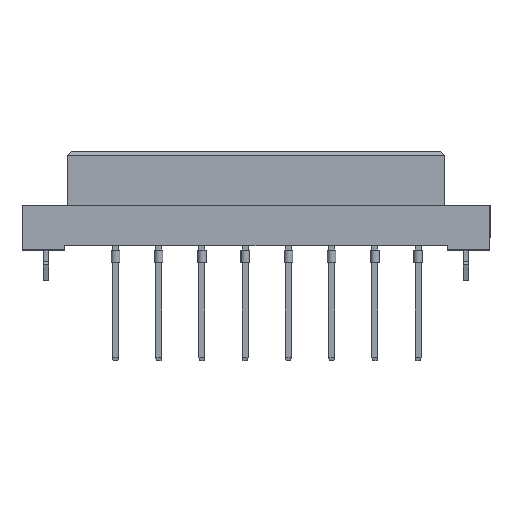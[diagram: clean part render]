
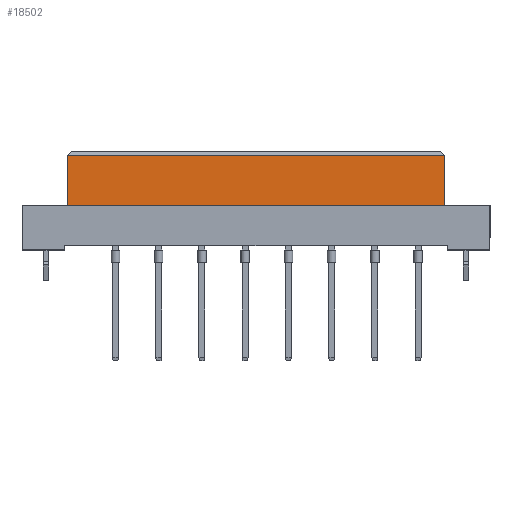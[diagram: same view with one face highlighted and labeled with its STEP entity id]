
A CAD part, top view. The second image highlights one B-rep face of the part: STEP entity #18502.
In plain terms, the highlighted planar face has unit normal (0, 0, 1).
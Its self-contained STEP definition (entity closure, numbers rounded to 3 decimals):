
#47 = ORIENTED_EDGE ( 'NONE', *, *, #4174, .T. ) ;
#268 = VERTEX_POINT ( 'NONE', #11756 ) ;
#723 = LINE ( 'NONE', #2539, #12637 ) ;
#931 = CARTESIAN_POINT ( 'NONE',  ( 22.2, -6.4, 4.25 ) ) ;
#2291 = EDGE_LOOP ( 'NONE', ( #14240, #47, #13957, #8863 ) ) ;
#2294 = AXIS2_PLACEMENT_3D ( 'NONE', #931, #10367, #7454 ) ;
#2538 = FACE_OUTER_BOUND ( 'NONE', #2291, .T. ) ;
#2539 = CARTESIAN_POINT ( 'NONE',  ( -22.2, -6.4, 4.25 ) ) ;
#2969 = CARTESIAN_POINT ( 'NONE',  ( 22.2, -6.4, 4.25 ) ) ;
#3035 = CARTESIAN_POINT ( 'NONE',  ( -22.2, -0.5, 4.25 ) ) ;
#3071 = LINE ( 'NONE', #2969, #4514 ) ;
#4174 = EDGE_CURVE ( 'NONE', #268, #17236, #5952, .T. ) ;
#4514 = VECTOR ( 'NONE', #11114, 1000. ) ;
#4851 = CARTESIAN_POINT ( 'NONE',  ( 22.2, -6.4, 4.25 ) ) ;
#5952 = LINE ( 'NONE', #18725, #11196 ) ;
#6397 = EDGE_CURVE ( 'NONE', #20586, #8257, #3071, .T. ) ;
#6808 = EDGE_CURVE ( 'NONE', #8257, #268, #15910, .T. ) ;
#7454 = DIRECTION ( 'NONE',  ( 1., 0., 0. ) ) ;
#8257 = VERTEX_POINT ( 'NONE', #15887 ) ;
#8863 = ORIENTED_EDGE ( 'NONE', *, *, #6397, .T. ) ;
#9249 = EDGE_CURVE ( 'NONE', #20586, #17236, #723, .T. ) ;
#10367 = DIRECTION ( 'NONE',  ( 0., 0., 1. ) ) ;
#11114 = DIRECTION ( 'NONE',  ( 1., 0., 0. ) ) ;
#11196 = VECTOR ( 'NONE', #17338, 1000. ) ;
#11301 = DIRECTION ( 'NONE',  ( 0., 1., 0. ) ) ;
#11756 = CARTESIAN_POINT ( 'NONE',  ( 22.2, -0.5, 4.25 ) ) ;
#12095 = VECTOR ( 'NONE', #11301, 1000. ) ;
#12637 = VECTOR ( 'NONE', #13916, 1000. ) ;
#13916 = DIRECTION ( 'NONE',  ( 0., 1., 0. ) ) ;
#13957 = ORIENTED_EDGE ( 'NONE', *, *, #9249, .F. ) ;
#14240 = ORIENTED_EDGE ( 'NONE', *, *, #6808, .T. ) ;
#15618 = PLANE ( 'NONE',  #2294 ) ;
#15887 = CARTESIAN_POINT ( 'NONE',  ( 22.2, -6.4, 4.25 ) ) ;
#15910 = LINE ( 'NONE', #4851, #12095 ) ;
#17087 = CARTESIAN_POINT ( 'NONE',  ( -22.2, -6.4, 4.25 ) ) ;
#17236 = VERTEX_POINT ( 'NONE', #3035 ) ;
#17338 = DIRECTION ( 'NONE',  ( -1., 0., 0. ) ) ;
#18502 = ADVANCED_FACE ( 'NONE', ( #2538 ), #15618, .T. ) ;
#18725 = CARTESIAN_POINT ( 'NONE',  ( -22.2, -0.5, 4.25 ) ) ;
#20586 = VERTEX_POINT ( 'NONE', #17087 ) ;
